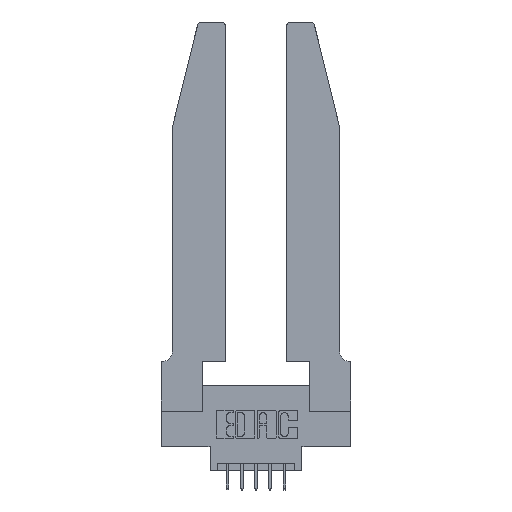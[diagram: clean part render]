
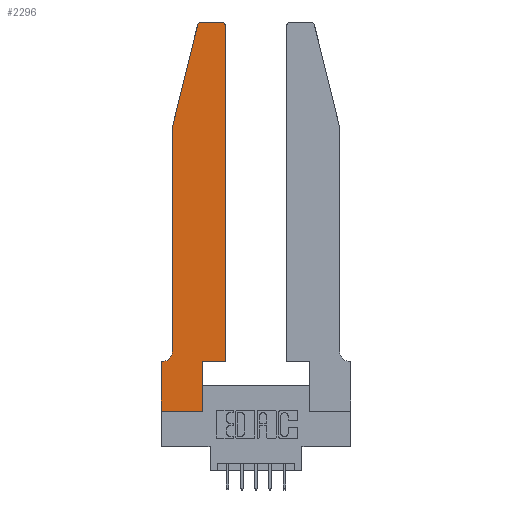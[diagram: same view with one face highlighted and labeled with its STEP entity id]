
A CAD part, top view. The second image highlights one B-rep face of the part: STEP entity #2296.
In plain terms, the highlighted planar face has unit normal (0, 0, 1).
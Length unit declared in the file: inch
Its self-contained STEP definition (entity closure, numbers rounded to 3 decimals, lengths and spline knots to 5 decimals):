
#10 = DIRECTION ( 'NONE',  ( 0., 0., 1. ) ) ;
#360 = EDGE_CURVE ( 'NONE', #6669, #10480, #4615, .T. ) ;
#614 = ORIENTED_EDGE ( 'NONE', *, *, #11904, .T. ) ;
#1088 = DIRECTION ( 'NONE',  ( 0., 1., 0. ) ) ;
#1110 = AXIS2_PLACEMENT_3D ( 'NONE', #2833, #2011, #3103 ) ;
#1148 = EDGE_CURVE ( 'NONE', #9086, #8050, #6665, .T. ) ;
#1185 = LINE ( 'NONE', #5425, #4756 ) ;
#1187 = VERTEX_POINT ( 'NONE', #6382 ) ;
#1268 = DIRECTION ( 'NONE',  ( 1., 0., 0. ) ) ;
#1444 = DIRECTION ( 'NONE',  ( -1., 0., 0. ) ) ;
#1574 = CARTESIAN_POINT ( 'NONE',  ( 0.2865, 0.35, 0.37 ) ) ;
#1838 = LINE ( 'NONE', #7295, #12299 ) ;
#1920 = CARTESIAN_POINT ( 'NONE',  ( 0.284, 2.75, 0.37 ) ) ;
#2011 = DIRECTION ( 'NONE',  ( 0., 0., 1. ) ) ;
#2296 = ADVANCED_FACE ( 'NONE', ( #7118 ), #12480, .T. ) ;
#2405 = CARTESIAN_POINT ( 'NONE',  ( 0.4505, 0.35, 0.37 ) ) ;
#2745 = EDGE_CURVE ( 'NONE', #12397, #11760, #7387, .T. ) ;
#2794 = ORIENTED_EDGE ( 'NONE', *, *, #360, .T. ) ;
#2833 = CARTESIAN_POINT ( 'NONE',  ( 0., 0.35, 0.37 ) ) ;
#2868 = ORIENTED_EDGE ( 'NONE', *, *, #1148, .T. ) ;
#2894 = CARTESIAN_POINT ( 'NONE',  ( 0.0755, 0.42, 0.37 ) ) ;
#3044 = CIRCLE ( 'NONE', #3950, 0.03 ) ;
#3103 = DIRECTION ( 'NONE',  ( 1., 0., 0. ) ) ;
#3331 = ORIENTED_EDGE ( 'NONE', *, *, #6728, .T. ) ;
#3406 = CARTESIAN_POINT ( 'NONE',  ( 0., 0.35, 0.37 ) ) ;
#3456 = DIRECTION ( 'NONE',  ( 1., 0., 0. ) ) ;
#3681 = ORIENTED_EDGE ( 'NONE', *, *, #4097, .T. ) ;
#3767 = VECTOR ( 'NONE', #3456, 39.37008 ) ;
#3825 = DIRECTION ( 'NONE',  ( 0., 0., 1. ) ) ;
#3950 = AXIS2_PLACEMENT_3D ( 'NONE', #8139, #10, #4256 ) ;
#4097 = EDGE_CURVE ( 'NONE', #5685, #9647, #6600, .T. ) ;
#4256 = DIRECTION ( 'NONE',  ( 1., 0., 0. ) ) ;
#4615 = CIRCLE ( 'NONE', #12488, 0.07 ) ;
#4679 = CARTESIAN_POINT ( 'NONE',  ( 0.4505, 0.35, 0.37 ) ) ;
#4756 = VECTOR ( 'NONE', #8401, 39.37008 ) ;
#4866 = ORIENTED_EDGE ( 'NONE', *, *, #8215, .T. ) ;
#5033 = EDGE_CURVE ( 'NONE', #7584, #9086, #5566, .T. ) ;
#5085 = CIRCLE ( 'NONE', #5757, 0.03 ) ;
#5425 = CARTESIAN_POINT ( 'NONE',  ( 0., 0., 0.37 ) ) ;
#5463 = ORIENTED_EDGE ( 'NONE', *, *, #2745, .T. ) ;
#5566 = LINE ( 'NONE', #13115, #3767 ) ;
#5685 = VERTEX_POINT ( 'NONE', #7563 ) ;
#5728 = VERTEX_POINT ( 'NONE', #3406 ) ;
#5757 = AXIS2_PLACEMENT_3D ( 'NONE', #8197, #3825, #11436 ) ;
#6038 = DIRECTION ( 'NONE',  ( -1., 0., 0. ) ) ;
#6382 = CARTESIAN_POINT ( 'NONE',  ( 0.4205, 2.75, 0.37 ) ) ;
#6600 = LINE ( 'NONE', #2405, #13682 ) ;
#6665 = LINE ( 'NONE', #12956, #10933 ) ;
#6669 = VERTEX_POINT ( 'NONE', #2894 ) ;
#6705 = LINE ( 'NONE', #4679, #8126 ) ;
#6728 = EDGE_CURVE ( 'NONE', #11760, #6669, #10698, .T. ) ;
#6742 = DIRECTION ( 'NONE',  ( 0., 1., 0. ) ) ;
#6982 = VECTOR ( 'NONE', #9675, 39.37008 ) ;
#7118 = FACE_OUTER_BOUND ( 'NONE', #12221, .T. ) ;
#7171 = ORIENTED_EDGE ( 'NONE', *, *, #11980, .T. ) ;
#7295 = CARTESIAN_POINT ( 'NONE',  ( 0.2605, 2.75, 0.37 ) ) ;
#7356 = LINE ( 'NONE', #11868, #6982 ) ;
#7381 = EDGE_CURVE ( 'NONE', #13216, #12397, #3044, .T. ) ;
#7387 = LINE ( 'NONE', #7603, #8496 ) ;
#7451 = DIRECTION ( 'NONE',  ( -0.239, -0.971, 0. ) ) ;
#7563 = CARTESIAN_POINT ( 'NONE',  ( 0.4505, 0.35, 0.37 ) ) ;
#7584 = VERTEX_POINT ( 'NONE', #12402 ) ;
#7603 = CARTESIAN_POINT ( 'NONE',  ( 0.0755, 2., 0.37 ) ) ;
#7604 = DIRECTION ( 'NONE',  ( 0., -1., 0. ) ) ;
#8015 = ORIENTED_EDGE ( 'NONE', *, *, #12178, .T. ) ;
#8050 = VERTEX_POINT ( 'NONE', #1574 ) ;
#8126 = VECTOR ( 'NONE', #1268, 39.37008 ) ;
#8136 = ORIENTED_EDGE ( 'NONE', *, *, #7381, .T. ) ;
#8139 = CARTESIAN_POINT ( 'NONE',  ( 0.284, 2.72, 0.37 ) ) ;
#8197 = CARTESIAN_POINT ( 'NONE',  ( 0.4205, 2.72, 0.37 ) ) ;
#8215 = EDGE_CURVE ( 'NONE', #1187, #13216, #1838, .T. ) ;
#8401 = DIRECTION ( 'NONE',  ( 0., -1., 0. ) ) ;
#8412 = CARTESIAN_POINT ( 'NONE',  ( 0.0055, 0.35, 0.37 ) ) ;
#8496 = VECTOR ( 'NONE', #7451, 39.37008 ) ;
#9086 = VERTEX_POINT ( 'NONE', #13869 ) ;
#9413 = EDGE_CURVE ( 'NONE', #9647, #1187, #5085, .T. ) ;
#9647 = VERTEX_POINT ( 'NONE', #13818 ) ;
#9675 = DIRECTION ( 'NONE',  ( -1., 0., 0. ) ) ;
#9761 = VECTOR ( 'NONE', #7604, 39.37008 ) ;
#10480 = VERTEX_POINT ( 'NONE', #8412 ) ;
#10564 = ORIENTED_EDGE ( 'NONE', *, *, #9413, .T. ) ;
#10698 = LINE ( 'NONE', #12962, #9761 ) ;
#10933 = VECTOR ( 'NONE', #1088, 39.37008 ) ;
#11054 = CARTESIAN_POINT ( 'NONE',  ( 0.0055, 0.42, 0.37 ) ) ;
#11189 = DIRECTION ( 'NONE',  ( 0., 0., -1. ) ) ;
#11413 = ORIENTED_EDGE ( 'NONE', *, *, #5033, .T. ) ;
#11436 = DIRECTION ( 'NONE',  ( 1., 0., 0. ) ) ;
#11680 = CARTESIAN_POINT ( 'NONE',  ( 0.25487, 2.72718, 0.37 ) ) ;
#11760 = VERTEX_POINT ( 'NONE', #12576 ) ;
#11868 = CARTESIAN_POINT ( 'NONE',  ( 0.0755, 0.35, 0.37 ) ) ;
#11904 = EDGE_CURVE ( 'NONE', #10480, #5728, #7356, .T. ) ;
#11980 = EDGE_CURVE ( 'NONE', #8050, #5685, #6705, .T. ) ;
#12178 = EDGE_CURVE ( 'NONE', #5728, #7584, #1185, .T. ) ;
#12221 = EDGE_LOOP ( 'NONE', ( #4866, #8136, #5463, #3331, #2794, #614, #8015, #11413, #2868, #7171, #3681, #10564 ) ) ;
#12299 = VECTOR ( 'NONE', #6038, 39.37008 ) ;
#12397 = VERTEX_POINT ( 'NONE', #11680 ) ;
#12402 = CARTESIAN_POINT ( 'NONE',  ( 0., 0., 0.37 ) ) ;
#12480 = PLANE ( 'NONE',  #1110 ) ;
#12488 = AXIS2_PLACEMENT_3D ( 'NONE', #11054, #11189, #1444 ) ;
#12576 = CARTESIAN_POINT ( 'NONE',  ( 0.0755, 2., 0.37 ) ) ;
#12956 = CARTESIAN_POINT ( 'NONE',  ( 0.2865, 0.35, 0.37 ) ) ;
#12962 = CARTESIAN_POINT ( 'NONE',  ( 0.0755, 2., 0.37 ) ) ;
#13115 = CARTESIAN_POINT ( 'NONE',  ( 0., 0., 0.37 ) ) ;
#13216 = VERTEX_POINT ( 'NONE', #1920 ) ;
#13682 = VECTOR ( 'NONE', #6742, 39.37008 ) ;
#13818 = CARTESIAN_POINT ( 'NONE',  ( 0.4505, 2.72, 0.37 ) ) ;
#13869 = CARTESIAN_POINT ( 'NONE',  ( 0.2865, 0., 0.37 ) ) ;
